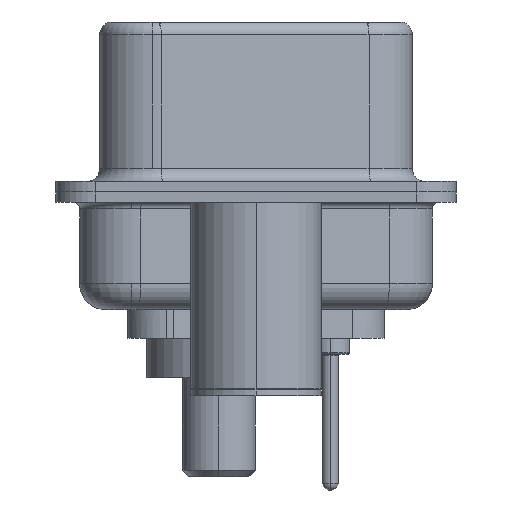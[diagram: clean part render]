
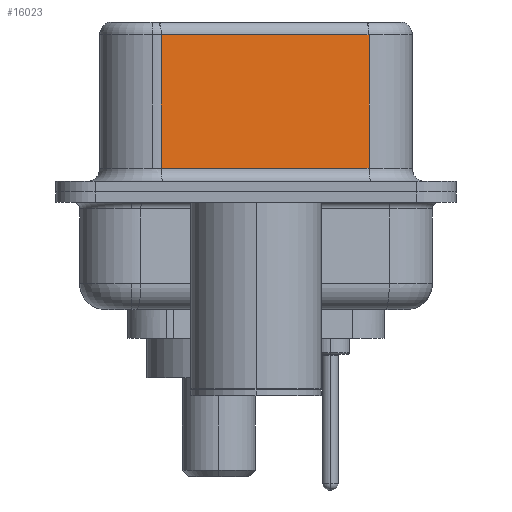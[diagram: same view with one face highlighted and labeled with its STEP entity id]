
A CAD part, left-side view. The second image highlights one B-rep face of the part: STEP entity #16023.
In plain terms, the highlighted planar face has unit normal (-0.985, -0.174, 0).
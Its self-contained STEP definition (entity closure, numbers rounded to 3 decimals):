
#936 = EDGE_CURVE ( 'NONE', #5498, #11724, #15851, .T. ) ;
#980 = LINE ( 'NONE', #8278, #9622 ) ;
#1216 = EDGE_LOOP ( 'NONE', ( #5815, #10869, #11227, #17542 ) ) ;
#1906 = CARTESIAN_POINT ( 'NONE',  ( 3.73, 3.628, 6.52 ) ) ;
#2666 = LINE ( 'NONE', #9488, #19582 ) ;
#3735 = VERTEX_POINT ( 'NONE', #15234 ) ;
#3865 = PLANE ( 'NONE',  #16982 ) ;
#4394 = VECTOR ( 'NONE', #19725, 1000. ) ;
#5481 = CARTESIAN_POINT ( 'NONE',  ( 3.73, 3.628, 6.02 ) ) ;
#5498 = VERTEX_POINT ( 'NONE', #5481 ) ;
#5815 = ORIENTED_EDGE ( 'NONE', *, *, #20828, .F. ) ;
#6079 = DIRECTION ( 'NONE',  ( -0.174, 0.985, 0. ) ) ;
#8113 = EDGE_CURVE ( 'NONE', #11724, #15287, #980, .T. ) ;
#8278 = CARTESIAN_POINT ( 'NONE',  ( 5.132, -4.322, 0.9 ) ) ;
#9087 = DIRECTION ( 'NONE',  ( -0.174, 0.985, 0. ) ) ;
#9488 = CARTESIAN_POINT ( 'NONE',  ( 5.132, -4.322, 6.02 ) ) ;
#9622 = VECTOR ( 'NONE', #21566, 1000. ) ;
#9738 = CARTESIAN_POINT ( 'NONE',  ( 5.132, -4.322, 6.52 ) ) ;
#10230 = FACE_OUTER_BOUND ( 'NONE', #1216, .T. ) ;
#10869 = ORIENTED_EDGE ( 'NONE', *, *, #17066, .T. ) ;
#11227 = ORIENTED_EDGE ( 'NONE', *, *, #936, .T. ) ;
#11402 = VECTOR ( 'NONE', #16766, 1000. ) ;
#11724 = VERTEX_POINT ( 'NONE', #12429 ) ;
#12345 = CARTESIAN_POINT ( 'NONE',  ( 5.132, -4.322, 6.52 ) ) ;
#12429 = CARTESIAN_POINT ( 'NONE',  ( 3.73, 3.628, 0.9 ) ) ;
#15234 = CARTESIAN_POINT ( 'NONE',  ( 5.132, -4.322, 6.02 ) ) ;
#15287 = VERTEX_POINT ( 'NONE', #20033 ) ;
#15851 = LINE ( 'NONE', #1906, #11402 ) ;
#16023 = ADVANCED_FACE ( 'NONE', ( #10230 ), #3865, .F. ) ;
#16766 = DIRECTION ( 'NONE',  ( 0., 0., -1. ) ) ;
#16982 = AXIS2_PLACEMENT_3D ( 'NONE', #12345, #19106, #9087 ) ;
#17066 = EDGE_CURVE ( 'NONE', #3735, #5498, #2666, .T. ) ;
#17542 = ORIENTED_EDGE ( 'NONE', *, *, #8113, .T. ) ;
#18392 = LINE ( 'NONE', #9738, #4394 ) ;
#19106 = DIRECTION ( 'NONE',  ( 0.985, 0.174, 0. ) ) ;
#19582 = VECTOR ( 'NONE', #6079, 1000. ) ;
#19725 = DIRECTION ( 'NONE',  ( 0., 0., -1. ) ) ;
#20033 = CARTESIAN_POINT ( 'NONE',  ( 5.132, -4.322, 0.9 ) ) ;
#20828 = EDGE_CURVE ( 'NONE', #3735, #15287, #18392, .T. ) ;
#21566 = DIRECTION ( 'NONE',  ( 0.174, -0.985, 0. ) ) ;
